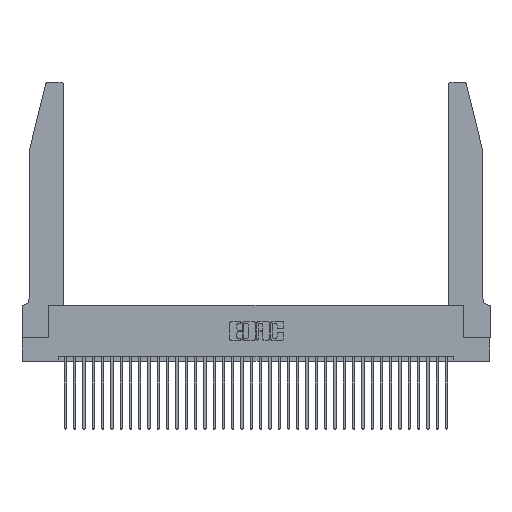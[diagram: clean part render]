
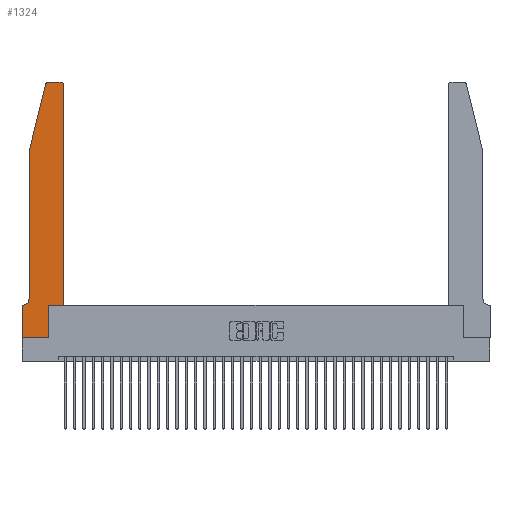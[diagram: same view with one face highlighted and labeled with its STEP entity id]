
A CAD part, top view. The second image highlights one B-rep face of the part: STEP entity #1324.
In plain terms, the highlighted planar face has unit normal (0, 0, 1).
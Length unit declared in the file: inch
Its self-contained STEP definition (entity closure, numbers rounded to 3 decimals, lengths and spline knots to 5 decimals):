
#173 = VECTOR ( 'NONE', #32837, 39.37008 ) ;
#648 = DIRECTION ( 'NONE',  ( 0., 1., 0. ) ) ;
#983 = LINE ( 'NONE', #29756, #6025 ) ;
#1240 = LINE ( 'NONE', #34342, #15421 ) ;
#1324 = ADVANCED_FACE ( 'NONE', ( #35158 ), #27257, .T. ) ;
#1679 = ORIENTED_EDGE ( 'NONE', *, *, #18270, .T. ) ;
#1854 = CARTESIAN_POINT ( 'NONE',  ( 0.2865, 0.35, 0.37 ) ) ;
#3328 = LINE ( 'NONE', #13295, #6998 ) ;
#3396 = LINE ( 'NONE', #21600, #23999 ) ;
#3692 = CARTESIAN_POINT ( 'NONE',  ( 0.2865, 0.35, 0.37 ) ) ;
#4349 = EDGE_CURVE ( 'NONE', #23924, #6871, #33631, .T. ) ;
#4523 = CIRCLE ( 'NONE', #22247, 0.03 ) ;
#4626 = CARTESIAN_POINT ( 'NONE',  ( 0.284, 2.75, 0.37 ) ) ;
#4756 = LINE ( 'NONE', #30395, #11233 ) ;
#4830 = DIRECTION ( 'NONE',  ( 0., 1., 0. ) ) ;
#5156 = CARTESIAN_POINT ( 'NONE',  ( 0.0055, 0.42, 0.37 ) ) ;
#5425 = LINE ( 'NONE', #3692, #10462 ) ;
#6025 = VECTOR ( 'NONE', #32462, 39.37008 ) ;
#6520 = VECTOR ( 'NONE', #23397, 39.37008 ) ;
#6871 = VERTEX_POINT ( 'NONE', #10511 ) ;
#6914 = EDGE_CURVE ( 'NONE', #27117, #35430, #15415, .T. ) ;
#6998 = VECTOR ( 'NONE', #10391, 39.37008 ) ;
#7070 = CARTESIAN_POINT ( 'NONE',  ( 0.0755, 2., 0.37 ) ) ;
#7241 = CARTESIAN_POINT ( 'NONE',  ( 0., 0., 0.37 ) ) ;
#7324 = ORIENTED_EDGE ( 'NONE', *, *, #18131, .T. ) ;
#7590 = ORIENTED_EDGE ( 'NONE', *, *, #6914, .T. ) ;
#7677 = DIRECTION ( 'NONE',  ( -1., 0., 0. ) ) ;
#8073 = AXIS2_PLACEMENT_3D ( 'NONE', #12120, #15157, #35556 ) ;
#9640 = EDGE_CURVE ( 'NONE', #6871, #12438, #3328, .T. ) ;
#9985 = EDGE_LOOP ( 'NONE', ( #7590, #11367, #21655, #12783, #24139, #24823, #20154, #7324, #11565, #1679, #22766, #23376 ) ) ;
#10391 = DIRECTION ( 'NONE',  ( -1., 0., 0. ) ) ;
#10462 = VECTOR ( 'NONE', #648, 39.37008 ) ;
#10511 = CARTESIAN_POINT ( 'NONE',  ( 0.0055, 0.35, 0.37 ) ) ;
#11233 = VECTOR ( 'NONE', #33461, 39.37008 ) ;
#11364 = VERTEX_POINT ( 'NONE', #7070 ) ;
#11367 = ORIENTED_EDGE ( 'NONE', *, *, #15317, .T. ) ;
#11565 = ORIENTED_EDGE ( 'NONE', *, *, #24096, .T. ) ;
#12120 = CARTESIAN_POINT ( 'NONE',  ( 0.4205, 2.72, 0.37 ) ) ;
#12438 = VERTEX_POINT ( 'NONE', #14069 ) ;
#12783 = ORIENTED_EDGE ( 'NONE', *, *, #34571, .T. ) ;
#12951 = DIRECTION ( 'NONE',  ( 1., 0., 0. ) ) ;
#13295 = CARTESIAN_POINT ( 'NONE',  ( 0.0755, 0.35, 0.37 ) ) ;
#13298 = DIRECTION ( 'NONE',  ( 1., 0., 0. ) ) ;
#14069 = CARTESIAN_POINT ( 'NONE',  ( 0., 0.35, 0.37 ) ) ;
#14242 = VERTEX_POINT ( 'NONE', #35970 ) ;
#14428 = CARTESIAN_POINT ( 'NONE',  ( 0.2865, 0., 0.37 ) ) ;
#15157 = DIRECTION ( 'NONE',  ( 0., 0., 1. ) ) ;
#15317 = EDGE_CURVE ( 'NONE', #35430, #14242, #4523, .T. ) ;
#15415 = LINE ( 'NONE', #16481, #34636 ) ;
#15421 = VECTOR ( 'NONE', #4830, 39.37008 ) ;
#15894 = CARTESIAN_POINT ( 'NONE',  ( 0.4505, 0.35, 0.37 ) ) ;
#16481 = CARTESIAN_POINT ( 'NONE',  ( 0.2605, 2.75, 0.37 ) ) ;
#17606 = AXIS2_PLACEMENT_3D ( 'NONE', #5156, #37167, #19735 ) ;
#18131 = EDGE_CURVE ( 'NONE', #31804, #19836, #4756, .T. ) ;
#18270 = EDGE_CURVE ( 'NONE', #29213, #27039, #3396, .T. ) ;
#18820 = DIRECTION ( 'NONE',  ( 0., 0., 1. ) ) ;
#18957 = CIRCLE ( 'NONE', #8073, 0.03 ) ;
#19735 = DIRECTION ( 'NONE',  ( -1., 0., 0. ) ) ;
#19836 = VERTEX_POINT ( 'NONE', #14428 ) ;
#20154 = ORIENTED_EDGE ( 'NONE', *, *, #35788, .T. ) ;
#21152 = LINE ( 'NONE', #35550, #6520 ) ;
#21600 = CARTESIAN_POINT ( 'NONE',  ( 0.4505, 0.35, 0.37 ) ) ;
#21627 = DIRECTION ( 'NONE',  ( 0., 0., 1. ) ) ;
#21655 = ORIENTED_EDGE ( 'NONE', *, *, #35031, .T. ) ;
#22247 = AXIS2_PLACEMENT_3D ( 'NONE', #33354, #18820, #25145 ) ;
#22766 = ORIENTED_EDGE ( 'NONE', *, *, #28454, .T. ) ;
#23376 = ORIENTED_EDGE ( 'NONE', *, *, #33911, .T. ) ;
#23397 = DIRECTION ( 'NONE',  ( -0.239, -0.971, 0. ) ) ;
#23924 = VERTEX_POINT ( 'NONE', #35814 ) ;
#23999 = VECTOR ( 'NONE', #13298, 39.37008 ) ;
#24096 = EDGE_CURVE ( 'NONE', #19836, #29213, #5425, .T. ) ;
#24139 = ORIENTED_EDGE ( 'NONE', *, *, #4349, .T. ) ;
#24823 = ORIENTED_EDGE ( 'NONE', *, *, #9640, .T. ) ;
#25145 = DIRECTION ( 'NONE',  ( 1., 0., 0. ) ) ;
#26863 = CARTESIAN_POINT ( 'NONE',  ( 0.0755, 2., 0.37 ) ) ;
#27039 = VERTEX_POINT ( 'NONE', #15894 ) ;
#27117 = VERTEX_POINT ( 'NONE', #31485 ) ;
#27257 = PLANE ( 'NONE',  #31483 ) ;
#28454 = EDGE_CURVE ( 'NONE', #27039, #28950, #1240, .T. ) ;
#28950 = VERTEX_POINT ( 'NONE', #35896 ) ;
#29213 = VERTEX_POINT ( 'NONE', #1854 ) ;
#29756 = CARTESIAN_POINT ( 'NONE',  ( 0., 0., 0.37 ) ) ;
#30395 = CARTESIAN_POINT ( 'NONE',  ( 0., 0., 0.37 ) ) ;
#31483 = AXIS2_PLACEMENT_3D ( 'NONE', #33220, #21627, #12951 ) ;
#31485 = CARTESIAN_POINT ( 'NONE',  ( 0.4205, 2.75, 0.37 ) ) ;
#31804 = VERTEX_POINT ( 'NONE', #7241 ) ;
#32462 = DIRECTION ( 'NONE',  ( 0., -1., 0. ) ) ;
#32837 = DIRECTION ( 'NONE',  ( 0., -1., 0. ) ) ;
#33220 = CARTESIAN_POINT ( 'NONE',  ( 0., 0.35, 0.37 ) ) ;
#33354 = CARTESIAN_POINT ( 'NONE',  ( 0.284, 2.72, 0.37 ) ) ;
#33461 = DIRECTION ( 'NONE',  ( 1., 0., 0. ) ) ;
#33631 = CIRCLE ( 'NONE', #17606, 0.07 ) ;
#33911 = EDGE_CURVE ( 'NONE', #28950, #27117, #18957, .T. ) ;
#34342 = CARTESIAN_POINT ( 'NONE',  ( 0.4505, 0.35, 0.37 ) ) ;
#34571 = EDGE_CURVE ( 'NONE', #11364, #23924, #34888, .T. ) ;
#34636 = VECTOR ( 'NONE', #7677, 39.37008 ) ;
#34888 = LINE ( 'NONE', #26863, #173 ) ;
#35031 = EDGE_CURVE ( 'NONE', #14242, #11364, #21152, .T. ) ;
#35158 = FACE_OUTER_BOUND ( 'NONE', #9985, .T. ) ;
#35430 = VERTEX_POINT ( 'NONE', #4626 ) ;
#35550 = CARTESIAN_POINT ( 'NONE',  ( 0.0755, 2., 0.37 ) ) ;
#35556 = DIRECTION ( 'NONE',  ( 1., 0., 0. ) ) ;
#35788 = EDGE_CURVE ( 'NONE', #12438, #31804, #983, .T. ) ;
#35814 = CARTESIAN_POINT ( 'NONE',  ( 0.0755, 0.42, 0.37 ) ) ;
#35896 = CARTESIAN_POINT ( 'NONE',  ( 0.4505, 2.72, 0.37 ) ) ;
#35970 = CARTESIAN_POINT ( 'NONE',  ( 0.25487, 2.72718, 0.37 ) ) ;
#37167 = DIRECTION ( 'NONE',  ( 0., 0., -1. ) ) ;
